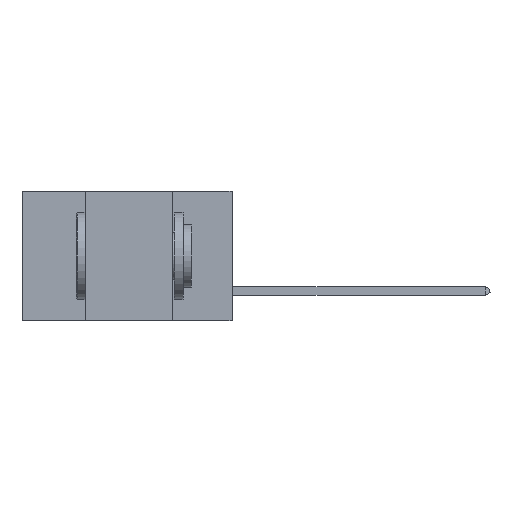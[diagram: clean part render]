
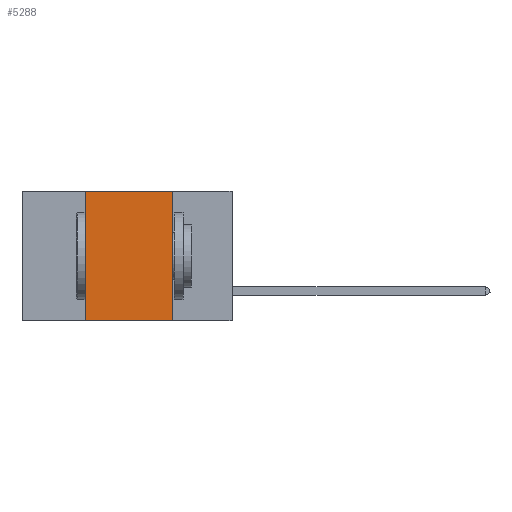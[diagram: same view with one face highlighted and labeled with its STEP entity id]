
A CAD part, left-side view. The second image highlights one B-rep face of the part: STEP entity #5288.
In plain terms, the highlighted planar face has unit normal (-1, 0, 0).
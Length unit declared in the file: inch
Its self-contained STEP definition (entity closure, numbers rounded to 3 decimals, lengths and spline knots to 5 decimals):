
#1082 = VERTEX_POINT ( 'NONE', #9940 ) ;
#1643 = ORIENTED_EDGE ( 'NONE', *, *, #2982, .F. ) ;
#1645 = VECTOR ( 'NONE', #11300, 39.37008 ) ;
#2982 = EDGE_CURVE ( 'NONE', #27335, #3180, #16927, .T. ) ;
#3180 = VERTEX_POINT ( 'NONE', #22873 ) ;
#3887 = CARTESIAN_POINT ( 'NONE',  ( 0., 0.6, 0. ) ) ;
#5167 = CARTESIAN_POINT ( 'NONE',  ( 0., 0.6, 0. ) ) ;
#5288 = ADVANCED_FACE ( 'NONE', ( #24064 ), #20064, .F. ) ;
#6287 = EDGE_CURVE ( 'NONE', #1082, #30870, #31845, .T. ) ;
#6664 = ORIENTED_EDGE ( 'NONE', *, *, #13212, .F. ) ;
#7340 = DIRECTION ( 'NONE',  ( 0., 0., -1. ) ) ;
#8259 = LINE ( 'NONE', #16389, #1645 ) ;
#9638 = CARTESIAN_POINT ( 'NONE',  ( 0., 0.17, 0. ) ) ;
#9940 = CARTESIAN_POINT ( 'NONE',  ( 0., 0.42, -0.37 ) ) ;
#10248 = VECTOR ( 'NONE', #21354, 39.37008 ) ;
#11300 = DIRECTION ( 'NONE',  ( 0., 0., 1. ) ) ;
#12121 = DIRECTION ( 'NONE',  ( 0., 0., -1. ) ) ;
#12429 = AXIS2_PLACEMENT_3D ( 'NONE', #5167, #22518, #12121 ) ;
#13212 = EDGE_CURVE ( 'NONE', #1082, #27335, #8259, .T. ) ;
#14434 = LINE ( 'NONE', #9638, #28522 ) ;
#16389 = CARTESIAN_POINT ( 'NONE',  ( 0., 0.42, 0. ) ) ;
#16927 = LINE ( 'NONE', #3887, #10248 ) ;
#19533 = EDGE_CURVE ( 'NONE', #3180, #30870, #14434, .T. ) ;
#19732 = CARTESIAN_POINT ( 'NONE',  ( 0., 0.6, -0.37 ) ) ;
#20064 = PLANE ( 'NONE',  #12429 ) ;
#21354 = DIRECTION ( 'NONE',  ( 0., -1., 0. ) ) ;
#22273 = DIRECTION ( 'NONE',  ( 0., -1., 0. ) ) ;
#22518 = DIRECTION ( 'NONE',  ( 1., 0., 0. ) ) ;
#22873 = CARTESIAN_POINT ( 'NONE',  ( 0., 0.17, 0. ) ) ;
#24064 = FACE_OUTER_BOUND ( 'NONE', #28199, .T. ) ;
#24372 = VECTOR ( 'NONE', #22273, 39.37008 ) ;
#24774 = ORIENTED_EDGE ( 'NONE', *, *, #19533, .F. ) ;
#25894 = CARTESIAN_POINT ( 'NONE',  ( 0., 0.17, -0.37 ) ) ;
#25963 = CARTESIAN_POINT ( 'NONE',  ( 0., 0.42, 0. ) ) ;
#27335 = VERTEX_POINT ( 'NONE', #25963 ) ;
#28199 = EDGE_LOOP ( 'NONE', ( #24774, #1643, #6664, #29520 ) ) ;
#28522 = VECTOR ( 'NONE', #7340, 39.37008 ) ;
#29520 = ORIENTED_EDGE ( 'NONE', *, *, #6287, .T. ) ;
#30870 = VERTEX_POINT ( 'NONE', #25894 ) ;
#31845 = LINE ( 'NONE', #19732, #24372 ) ;
